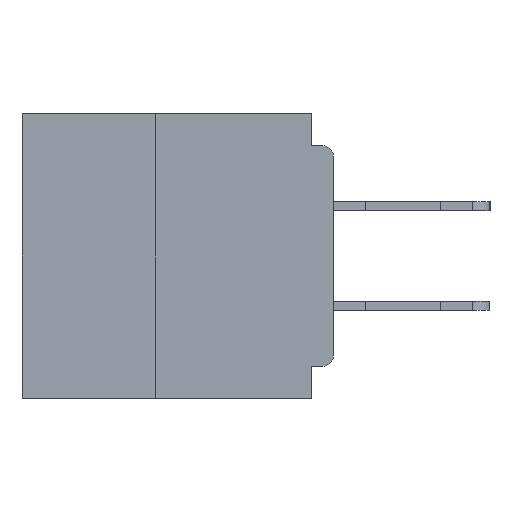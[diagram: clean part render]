
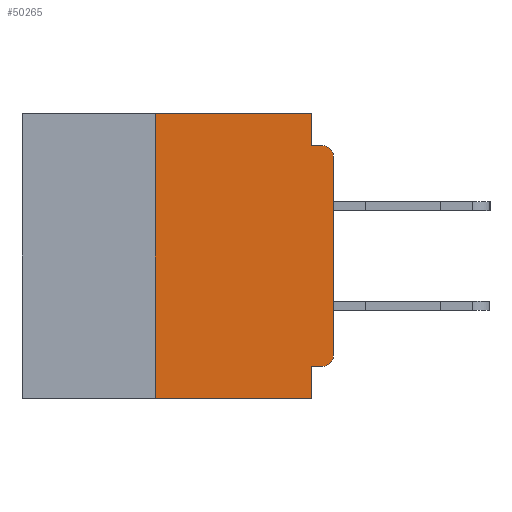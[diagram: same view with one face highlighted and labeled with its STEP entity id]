
A CAD part, left-side view. The second image highlights one B-rep face of the part: STEP entity #50265.
In plain terms, the highlighted planar face has unit normal (-1, 0, 0).
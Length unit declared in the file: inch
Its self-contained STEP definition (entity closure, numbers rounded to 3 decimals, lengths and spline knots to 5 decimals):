
#511 = VECTOR ( 'NONE', #15578, 39.37008 ) ;
#809 = LINE ( 'NONE', #38280, #50934 ) ;
#1465 = CARTESIAN_POINT ( 'NONE',  ( 0., 0., 0. ) ) ;
#1802 = FACE_OUTER_BOUND ( 'NONE', #15799, .T. ) ;
#2680 = DIRECTION ( 'NONE',  ( 0., 0., -1. ) ) ;
#2702 = EDGE_CURVE ( 'NONE', #32105, #45059, #31138, .T. ) ;
#4168 = CARTESIAN_POINT ( 'NONE',  ( 0., 0.031, -0.045 ) ) ;
#4511 = VERTEX_POINT ( 'NONE', #32392 ) ;
#5452 = VECTOR ( 'NONE', #6003, 39.37008 ) ;
#6003 = DIRECTION ( 'NONE',  ( 0., 0., -1. ) ) ;
#6204 = ORIENTED_EDGE ( 'NONE', *, *, #19192, .F. ) ;
#7164 = VERTEX_POINT ( 'NONE', #34828 ) ;
#7469 = DIRECTION ( 'NONE',  ( 0., 1., 0. ) ) ;
#7797 = AXIS2_PLACEMENT_3D ( 'NONE', #29488, #37577, #13893 ) ;
#7937 = CARTESIAN_POINT ( 'NONE',  ( 0., 0.015, -0.34 ) ) ;
#9668 = VERTEX_POINT ( 'NONE', #4168 ) ;
#10652 = VECTOR ( 'NONE', #41181, 39.37008 ) ;
#11908 = LINE ( 'NONE', #1465, #10652 ) ;
#11941 = CARTESIAN_POINT ( 'NONE',  ( 0., 0.437, 0. ) ) ;
#11967 = DIRECTION ( 'NONE',  ( 0., 0., -1. ) ) ;
#12897 = CARTESIAN_POINT ( 'NONE',  ( 0., 0.015, -0.355 ) ) ;
#13407 = AXIS2_PLACEMENT_3D ( 'NONE', #7937, #35637, #11967 ) ;
#13893 = DIRECTION ( 'NONE',  ( 0., 0., -1. ) ) ;
#14449 = CARTESIAN_POINT ( 'NONE',  ( 0., 0.031, 0. ) ) ;
#14659 = DIRECTION ( 'NONE',  ( 0., 0., 1. ) ) ;
#15578 = DIRECTION ( 'NONE',  ( 0., -1., 0. ) ) ;
#15734 = EDGE_CURVE ( 'NONE', #32105, #7164, #47884, .T. ) ;
#15799 = EDGE_LOOP ( 'NONE', ( #23004, #25440, #47638, #18693, #19913, #34081, #44582, #6204, #37817, #20562 ) ) ;
#16714 = CARTESIAN_POINT ( 'NONE',  ( 0., 0.25, -0.4 ) ) ;
#17617 = CARTESIAN_POINT ( 'NONE',  ( 0., 0.25, -0.4 ) ) ;
#17939 = AXIS2_PLACEMENT_3D ( 'NONE', #50071, #26491, #2680 ) ;
#18242 = EDGE_CURVE ( 'NONE', #38631, #45292, #31566, .T. ) ;
#18693 = ORIENTED_EDGE ( 'NONE', *, *, #38775, .F. ) ;
#18861 = DIRECTION ( 'NONE',  ( 0., -1., 0. ) ) ;
#19192 = EDGE_CURVE ( 'NONE', #45292, #7164, #26598, .T. ) ;
#19913 = ORIENTED_EDGE ( 'NONE', *, *, #25889, .F. ) ;
#20562 = ORIENTED_EDGE ( 'NONE', *, *, #41196, .T. ) ;
#21028 = LINE ( 'NONE', #14449, #51173 ) ;
#22634 = CIRCLE ( 'NONE', #13407, 0.015 ) ;
#22978 = LINE ( 'NONE', #11941, #511 ) ;
#23004 = ORIENTED_EDGE ( 'NONE', *, *, #37581, .T. ) ;
#25440 = ORIENTED_EDGE ( 'NONE', *, *, #35937, .T. ) ;
#25693 = VECTOR ( 'NONE', #18861, 39.37008 ) ;
#25889 = EDGE_CURVE ( 'NONE', #45059, #48485, #22978, .T. ) ;
#26491 = DIRECTION ( 'NONE',  ( -1., 0., 0. ) ) ;
#26598 = LINE ( 'NONE', #49229, #5452 ) ;
#26975 = CARTESIAN_POINT ( 'NONE',  ( 0., 0.031, -0.355 ) ) ;
#27247 = CARTESIAN_POINT ( 'NONE',  ( 0., 0., -0.355 ) ) ;
#28889 = CARTESIAN_POINT ( 'NONE',  ( 0., 0.25, 0. ) ) ;
#29488 = CARTESIAN_POINT ( 'NONE',  ( 0., 0.437, 0. ) ) ;
#30214 = DIRECTION ( 'NONE',  ( 0., 0., -1. ) ) ;
#31138 = LINE ( 'NONE', #16714, #50834 ) ;
#31566 = LINE ( 'NONE', #27247, #51269 ) ;
#32105 = VERTEX_POINT ( 'NONE', #17617 ) ;
#32392 = CARTESIAN_POINT ( 'NONE',  ( 0., 0., -0.34 ) ) ;
#33569 = PLANE ( 'NONE',  #7797 ) ;
#34081 = ORIENTED_EDGE ( 'NONE', *, *, #2702, .F. ) ;
#34828 = CARTESIAN_POINT ( 'NONE',  ( 0., 0.031, -0.4 ) ) ;
#34959 = CIRCLE ( 'NONE', #17939, 0.015 ) ;
#35637 = DIRECTION ( 'NONE',  ( -1., 0., 0. ) ) ;
#35937 = EDGE_CURVE ( 'NONE', #45242, #44919, #34959, .T. ) ;
#37577 = DIRECTION ( 'NONE',  ( 1., 0., 0. ) ) ;
#37581 = EDGE_CURVE ( 'NONE', #4511, #45242, #11908, .T. ) ;
#37817 = ORIENTED_EDGE ( 'NONE', *, *, #18242, .F. ) ;
#38280 = CARTESIAN_POINT ( 'NONE',  ( 0., 0., -0.045 ) ) ;
#38516 = CARTESIAN_POINT ( 'NONE',  ( 0., 0.437, -0.4 ) ) ;
#38631 = VERTEX_POINT ( 'NONE', #12897 ) ;
#38775 = EDGE_CURVE ( 'NONE', #48485, #9668, #21028, .T. ) ;
#40992 = EDGE_CURVE ( 'NONE', #9668, #44919, #809, .T. ) ;
#41181 = DIRECTION ( 'NONE',  ( 0., 0., 1. ) ) ;
#41196 = EDGE_CURVE ( 'NONE', #38631, #4511, #22634, .T. ) ;
#43908 = CARTESIAN_POINT ( 'NONE',  ( 0., 0.015, -0.045 ) ) ;
#44128 = CARTESIAN_POINT ( 'NONE',  ( 0., 0.031, 0. ) ) ;
#44582 = ORIENTED_EDGE ( 'NONE', *, *, #15734, .T. ) ;
#44919 = VERTEX_POINT ( 'NONE', #43908 ) ;
#45059 = VERTEX_POINT ( 'NONE', #28889 ) ;
#45242 = VERTEX_POINT ( 'NONE', #45792 ) ;
#45292 = VERTEX_POINT ( 'NONE', #26975 ) ;
#45792 = CARTESIAN_POINT ( 'NONE',  ( 0., 0., -0.06 ) ) ;
#47638 = ORIENTED_EDGE ( 'NONE', *, *, #40992, .F. ) ;
#47884 = LINE ( 'NONE', #38516, #25693 ) ;
#48485 = VERTEX_POINT ( 'NONE', #44128 ) ;
#49229 = CARTESIAN_POINT ( 'NONE',  ( 0., 0.031, -0.4 ) ) ;
#50071 = CARTESIAN_POINT ( 'NONE',  ( 0., 0.015, -0.06 ) ) ;
#50108 = DIRECTION ( 'NONE',  ( 0., -1., 0. ) ) ;
#50265 = ADVANCED_FACE ( 'NONE', ( #1802 ), #33569, .F. ) ;
#50834 = VECTOR ( 'NONE', #14659, 39.37008 ) ;
#50934 = VECTOR ( 'NONE', #50108, 39.37008 ) ;
#51173 = VECTOR ( 'NONE', #30214, 39.37008 ) ;
#51269 = VECTOR ( 'NONE', #7469, 39.37008 ) ;
